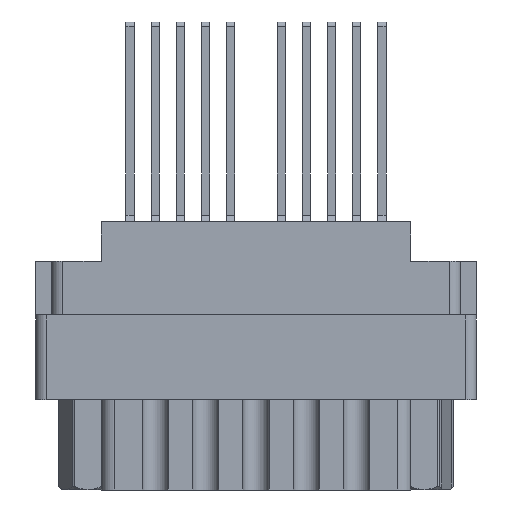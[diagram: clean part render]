
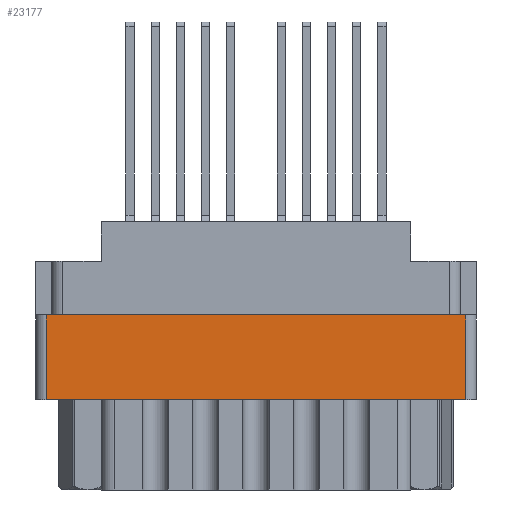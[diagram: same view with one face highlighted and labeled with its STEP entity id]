
A CAD part, front view. The second image highlights one B-rep face of the part: STEP entity #23177.
In plain terms, the highlighted planar face has unit normal (0, -1, 0).
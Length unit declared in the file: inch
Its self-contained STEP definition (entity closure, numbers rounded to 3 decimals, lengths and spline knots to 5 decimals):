
#2094 = EDGE_CURVE ( 'NONE', #14928, #4619, #27256, .T. ) ;
#2465 = ORIENTED_EDGE ( 'NONE', *, *, #2094, .F. ) ;
#2903 = VECTOR ( 'NONE', #36773, 39.37008 ) ;
#2946 = DIRECTION ( 'NONE',  ( 0., 0., 1. ) ) ;
#3472 = EDGE_CURVE ( 'NONE', #6958, #4619, #23566, .T. ) ;
#4619 = VERTEX_POINT ( 'NONE', #24646 ) ;
#4911 = CARTESIAN_POINT ( 'NONE',  ( -0.624, -0.343, -0.798 ) ) ;
#6958 = VERTEX_POINT ( 'NONE', #22331 ) ;
#8185 = DIRECTION ( 'NONE',  ( -1., 0., 0. ) ) ;
#8974 = FACE_OUTER_BOUND ( 'NONE', #28201, .T. ) ;
#9623 = ORIENTED_EDGE ( 'NONE', *, *, #20955, .T. ) ;
#9969 = VECTOR ( 'NONE', #8185, 39.37008 ) ;
#12055 = EDGE_CURVE ( 'NONE', #6958, #36691, #17574, .T. ) ;
#12516 = AXIS2_PLACEMENT_3D ( 'NONE', #35757, #13129, #15643 ) ;
#13129 = DIRECTION ( 'NONE',  ( 0., -1., 0. ) ) ;
#13215 = CARTESIAN_POINT ( 'NONE',  ( -0.624, -0.343, -0.529 ) ) ;
#14928 = VERTEX_POINT ( 'NONE', #27486 ) ;
#15643 = DIRECTION ( 'NONE',  ( 0., 0., -1. ) ) ;
#17574 = LINE ( 'NONE', #19438, #9969 ) ;
#17830 = VECTOR ( 'NONE', #23682, 39.37008 ) ;
#19438 = CARTESIAN_POINT ( 'NONE',  ( 0., -0.343, -0.529 ) ) ;
#20955 = EDGE_CURVE ( 'NONE', #14928, #36691, #33834, .T. ) ;
#21398 = ORIENTED_EDGE ( 'NONE', *, *, #3472, .T. ) ;
#22331 = CARTESIAN_POINT ( 'NONE',  ( 0.624, -0.343, -0.529 ) ) ;
#22978 = CARTESIAN_POINT ( 'NONE',  ( 0.624, -0.343, -0.798 ) ) ;
#23177 = ADVANCED_FACE ( 'NONE', ( #8974 ), #30209, .T. ) ;
#23222 = ORIENTED_EDGE ( 'NONE', *, *, #12055, .F. ) ;
#23566 = LINE ( 'NONE', #22978, #35728 ) ;
#23682 = DIRECTION ( 'NONE',  ( 1., 0., 0. ) ) ;
#24646 = CARTESIAN_POINT ( 'NONE',  ( 0.624, -0.343, -0.277 ) ) ;
#26699 = CARTESIAN_POINT ( 'NONE',  ( 0., -0.343, -0.277 ) ) ;
#27256 = LINE ( 'NONE', #26699, #17830 ) ;
#27486 = CARTESIAN_POINT ( 'NONE',  ( -0.624, -0.343, -0.277 ) ) ;
#28201 = EDGE_LOOP ( 'NONE', ( #2465, #9623, #23222, #21398 ) ) ;
#30209 = PLANE ( 'NONE',  #12516 ) ;
#33834 = LINE ( 'NONE', #4911, #2903 ) ;
#35728 = VECTOR ( 'NONE', #2946, 39.37008 ) ;
#35757 = CARTESIAN_POINT ( 'NONE',  ( -0.656, -0.343, -0.798 ) ) ;
#36691 = VERTEX_POINT ( 'NONE', #13215 ) ;
#36773 = DIRECTION ( 'NONE',  ( 0., 0., -1. ) ) ;
